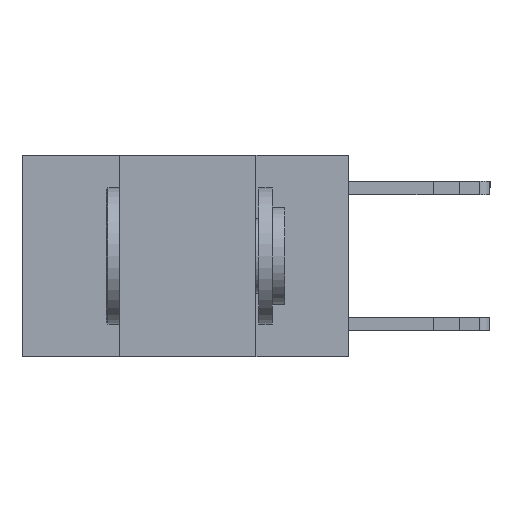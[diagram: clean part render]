
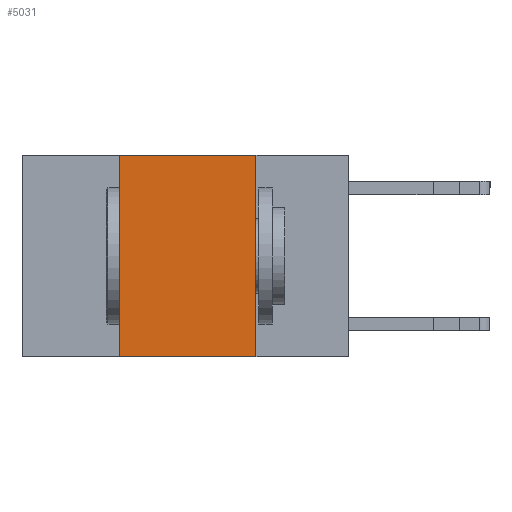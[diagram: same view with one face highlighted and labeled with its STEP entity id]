
A CAD part, left-side view. The second image highlights one B-rep face of the part: STEP entity #5031.
In plain terms, the highlighted planar face has unit normal (-1, 0, 0).
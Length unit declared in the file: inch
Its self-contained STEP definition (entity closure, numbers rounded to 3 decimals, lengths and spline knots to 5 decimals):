
#121 = LINE ( 'NONE', #4890, #8718 ) ;
#450 = FACE_OUTER_BOUND ( 'NONE', #941, .T. ) ;
#941 = EDGE_LOOP ( 'NONE', ( #13317, #4557, #13744, #12349 ) ) ;
#1071 = CARTESIAN_POINT ( 'NONE',  ( 0., 0.6, 0. ) ) ;
#3352 = CARTESIAN_POINT ( 'NONE',  ( 0., 0.17, -0.37 ) ) ;
#3765 = VERTEX_POINT ( 'NONE', #9547 ) ;
#4325 = VERTEX_POINT ( 'NONE', #3352 ) ;
#4557 = ORIENTED_EDGE ( 'NONE', *, *, #6262, .F. ) ;
#4890 = CARTESIAN_POINT ( 'NONE',  ( 0., 0.17, 0. ) ) ;
#4897 = EDGE_CURVE ( 'NONE', #15625, #4325, #121, .T. ) ;
#5004 = VECTOR ( 'NONE', #5377, 39.37008 ) ;
#5031 = ADVANCED_FACE ( 'NONE', ( #450 ), #13028, .F. ) ;
#5227 = DIRECTION ( 'NONE',  ( 0., 0., -1. ) ) ;
#5377 = DIRECTION ( 'NONE',  ( 0., -1., 0. ) ) ;
#5883 = EDGE_CURVE ( 'NONE', #6447, #4325, #7662, .T. ) ;
#6076 = DIRECTION ( 'NONE',  ( 0., -1., 0. ) ) ;
#6262 = EDGE_CURVE ( 'NONE', #3765, #15625, #13494, .T. ) ;
#6447 = VERTEX_POINT ( 'NONE', #13073 ) ;
#6636 = LINE ( 'NONE', #10735, #13255 ) ;
#6768 = DIRECTION ( 'NONE',  ( 1., 0., 0. ) ) ;
#7662 = LINE ( 'NONE', #10291, #5004 ) ;
#8718 = VECTOR ( 'NONE', #5227, 39.37008 ) ;
#9395 = DIRECTION ( 'NONE',  ( 0., 0., -1. ) ) ;
#9547 = CARTESIAN_POINT ( 'NONE',  ( 0., 0.42, 0. ) ) ;
#10291 = CARTESIAN_POINT ( 'NONE',  ( 0., 0.6, -0.37 ) ) ;
#10347 = CARTESIAN_POINT ( 'NONE',  ( 0., 0.17, 0. ) ) ;
#10735 = CARTESIAN_POINT ( 'NONE',  ( 0., 0.42, 0. ) ) ;
#12349 = ORIENTED_EDGE ( 'NONE', *, *, #5883, .T. ) ;
#12689 = VECTOR ( 'NONE', #6076, 39.37008 ) ;
#13028 = PLANE ( 'NONE',  #15321 ) ;
#13073 = CARTESIAN_POINT ( 'NONE',  ( 0., 0.42, -0.37 ) ) ;
#13255 = VECTOR ( 'NONE', #15754, 39.37008 ) ;
#13317 = ORIENTED_EDGE ( 'NONE', *, *, #4897, .F. ) ;
#13494 = LINE ( 'NONE', #1071, #12689 ) ;
#13744 = ORIENTED_EDGE ( 'NONE', *, *, #15767, .F. ) ;
#14338 = CARTESIAN_POINT ( 'NONE',  ( 0., 0.6, 0. ) ) ;
#15321 = AXIS2_PLACEMENT_3D ( 'NONE', #14338, #6768, #9395 ) ;
#15625 = VERTEX_POINT ( 'NONE', #10347 ) ;
#15754 = DIRECTION ( 'NONE',  ( 0., 0., 1. ) ) ;
#15767 = EDGE_CURVE ( 'NONE', #6447, #3765, #6636, .T. ) ;
